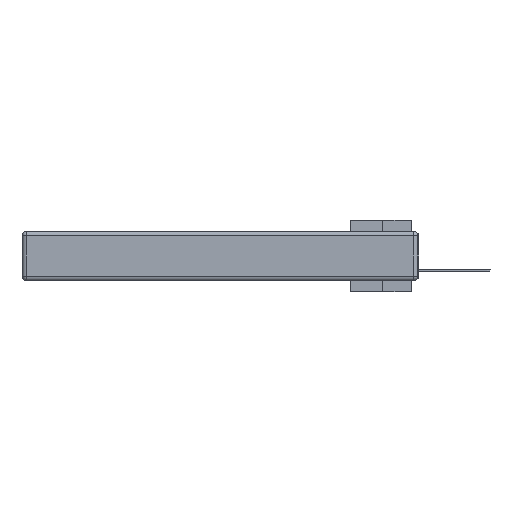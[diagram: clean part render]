
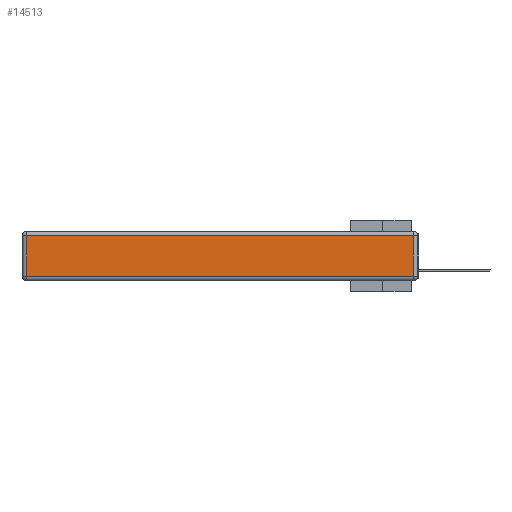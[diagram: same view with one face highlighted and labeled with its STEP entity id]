
A CAD part, left-side view. The second image highlights one B-rep face of the part: STEP entity #14513.
In plain terms, the highlighted planar face has unit normal (-1, 0, 0).
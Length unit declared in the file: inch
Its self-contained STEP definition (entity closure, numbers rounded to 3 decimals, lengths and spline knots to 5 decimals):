
#883 = EDGE_LOOP ( 'NONE', ( #14705, #18862, #20643, #1357 ) ) ;
#993 = PLANE ( 'NONE',  #11896 ) ;
#1357 = ORIENTED_EDGE ( 'NONE', *, *, #27031, .T. ) ;
#1983 = CARTESIAN_POINT ( 'NONE',  ( 0., 2.75, -0.03 ) ) ;
#2254 = CARTESIAN_POINT ( 'NONE',  ( 0., 2.72, -0.03 ) ) ;
#2433 = LINE ( 'NONE', #1983, #25270 ) ;
#2768 = CARTESIAN_POINT ( 'NONE',  ( 0., 2.72, -0.343 ) ) ;
#3378 = VECTOR ( 'NONE', #24747, 39.37008 ) ;
#4506 = CARTESIAN_POINT ( 'NONE',  ( 0., 2.72, -0.313 ) ) ;
#8862 = LINE ( 'NONE', #32729, #3378 ) ;
#11896 = AXIS2_PLACEMENT_3D ( 'NONE', #30889, #33594, #22632 ) ;
#12774 = VERTEX_POINT ( 'NONE', #2254 ) ;
#14513 = ADVANCED_FACE ( 'NONE', ( #28135 ), #993, .T. ) ;
#14705 = ORIENTED_EDGE ( 'NONE', *, *, #33306, .T. ) ;
#14990 = CARTESIAN_POINT ( 'NONE',  ( 0., 0., -0.313 ) ) ;
#14995 = VECTOR ( 'NONE', #24422, 39.37008 ) ;
#16358 = CARTESIAN_POINT ( 'NONE',  ( 0., 0.03, -0.03 ) ) ;
#18862 = ORIENTED_EDGE ( 'NONE', *, *, #23612, .T. ) ;
#20643 = ORIENTED_EDGE ( 'NONE', *, *, #24762, .T. ) ;
#22632 = DIRECTION ( 'NONE',  ( 0., 0., 1. ) ) ;
#23192 = VECTOR ( 'NONE', #25759, 39.37008 ) ;
#23612 = EDGE_CURVE ( 'NONE', #23861, #32397, #8862, .T. ) ;
#23861 = VERTEX_POINT ( 'NONE', #25793 ) ;
#24422 = DIRECTION ( 'NONE',  ( 0., 0., -1. ) ) ;
#24747 = DIRECTION ( 'NONE',  ( 0., 0., 1. ) ) ;
#24762 = EDGE_CURVE ( 'NONE', #32397, #12774, #2433, .T. ) ;
#25270 = VECTOR ( 'NONE', #34451, 39.37008 ) ;
#25759 = DIRECTION ( 'NONE',  ( 0., -1., 0. ) ) ;
#25793 = CARTESIAN_POINT ( 'NONE',  ( 0., 0.03, -0.313 ) ) ;
#27031 = EDGE_CURVE ( 'NONE', #12774, #31080, #34839, .T. ) ;
#28135 = FACE_OUTER_BOUND ( 'NONE', #883, .T. ) ;
#30386 = LINE ( 'NONE', #14990, #23192 ) ;
#30889 = CARTESIAN_POINT ( 'NONE',  ( 0., 0., -0.343 ) ) ;
#31080 = VERTEX_POINT ( 'NONE', #4506 ) ;
#32397 = VERTEX_POINT ( 'NONE', #16358 ) ;
#32729 = CARTESIAN_POINT ( 'NONE',  ( 0., 0.03, -0.343 ) ) ;
#33306 = EDGE_CURVE ( 'NONE', #31080, #23861, #30386, .T. ) ;
#33594 = DIRECTION ( 'NONE',  ( -1., 0., 0. ) ) ;
#34451 = DIRECTION ( 'NONE',  ( 0., 1., 0. ) ) ;
#34839 = LINE ( 'NONE', #2768, #14995 ) ;
